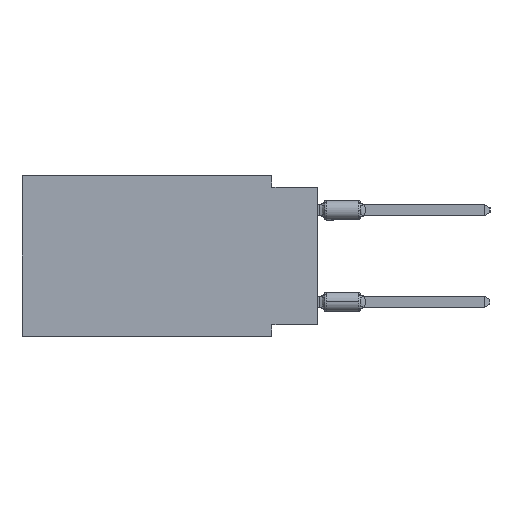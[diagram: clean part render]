
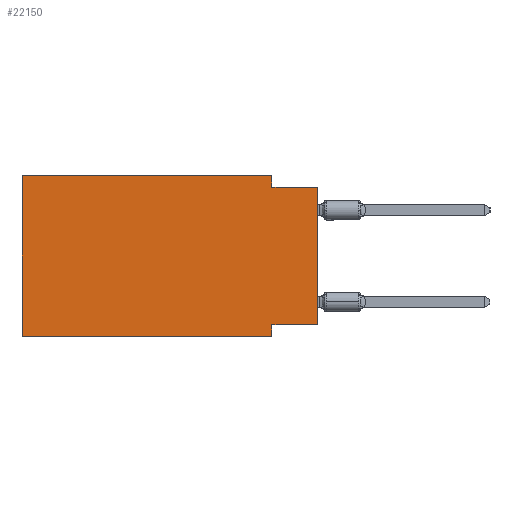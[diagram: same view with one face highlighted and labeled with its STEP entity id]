
A CAD part, left-side view. The second image highlights one B-rep face of the part: STEP entity #22150.
In plain terms, the highlighted planar face has unit normal (-1, 0, 0).
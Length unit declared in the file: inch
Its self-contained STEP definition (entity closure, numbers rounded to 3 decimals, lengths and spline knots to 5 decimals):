
#158 = ORIENTED_EDGE ( 'NONE', *, *, #56466, .F. ) ;
#306 = VECTOR ( 'NONE', #60173, 39.37008 ) ;
#511 = ORIENTED_EDGE ( 'NONE', *, *, #33676, .F. ) ;
#814 = DIRECTION ( 'NONE',  ( 0., 0., -1. ) ) ;
#1471 = VERTEX_POINT ( 'NONE', #30181 ) ;
#1937 = VECTOR ( 'NONE', #21164, 39.37008 ) ;
#1983 = CARTESIAN_POINT ( 'NONE',  ( 0., 0., -0.025 ) ) ;
#2095 = VECTOR ( 'NONE', #48235, 39.37008 ) ;
#4401 = VERTEX_POINT ( 'NONE', #27706 ) ;
#5204 = LINE ( 'NONE', #50768, #1937 ) ;
#7165 = LINE ( 'NONE', #27428, #7428 ) ;
#7428 = VECTOR ( 'NONE', #26779, 39.37008 ) ;
#8396 = CARTESIAN_POINT ( 'NONE',  ( 0., 0.645, -0.35 ) ) ;
#8616 = FACE_OUTER_BOUND ( 'NONE', #26243, .T. ) ;
#9308 = CARTESIAN_POINT ( 'NONE',  ( 0., 0.1, -0.325 ) ) ;
#11739 = CARTESIAN_POINT ( 'NONE',  ( 0., 0.1, -0.35 ) ) ;
#12294 = DIRECTION ( 'NONE',  ( 0., 0., -1. ) ) ;
#12541 = EDGE_CURVE ( 'NONE', #60988, #54172, #38979, .T. ) ;
#17719 = CARTESIAN_POINT ( 'NONE',  ( 0., 0.645, 0. ) ) ;
#18236 = LINE ( 'NONE', #63796, #39655 ) ;
#18323 = EDGE_CURVE ( 'NONE', #4401, #53427, #36437, .T. ) ;
#21164 = DIRECTION ( 'NONE',  ( 0., -1., 0. ) ) ;
#21546 = ORIENTED_EDGE ( 'NONE', *, *, #18323, .T. ) ;
#22150 = ADVANCED_FACE ( 'NONE', ( #8616 ), #28557, .F. ) ;
#23129 = VECTOR ( 'NONE', #27672, 39.37008 ) ;
#23740 = CARTESIAN_POINT ( 'NONE',  ( 0., 0.645, 0. ) ) ;
#26243 = EDGE_LOOP ( 'NONE', ( #21546, #32283, #41343, #34098, #158, #36931, #511, #52017 ) ) ;
#26779 = DIRECTION ( 'NONE',  ( 0., 1., 0. ) ) ;
#26961 = LINE ( 'NONE', #47257, #2095 ) ;
#27082 = DIRECTION ( 'NONE',  ( 0., 0., 1. ) ) ;
#27428 = CARTESIAN_POINT ( 'NONE',  ( 0., 0., -0.325 ) ) ;
#27672 = DIRECTION ( 'NONE',  ( 0., -1., 0. ) ) ;
#27706 = CARTESIAN_POINT ( 'NONE',  ( 0., 0., -0.325 ) ) ;
#28557 = PLANE ( 'NONE',  #49572 ) ;
#28885 = CARTESIAN_POINT ( 'NONE',  ( 0., 0.645, 0. ) ) ;
#29329 = CARTESIAN_POINT ( 'NONE',  ( 0., 0.1, -0.025 ) ) ;
#30181 = CARTESIAN_POINT ( 'NONE',  ( 0., 0.1, 0. ) ) ;
#30734 = LINE ( 'NONE', #46375, #46731 ) ;
#32283 = ORIENTED_EDGE ( 'NONE', *, *, #32775, .F. ) ;
#32775 = EDGE_CURVE ( 'NONE', #55610, #53427, #5204, .T. ) ;
#33571 = EDGE_CURVE ( 'NONE', #4401, #48348, #7165, .T. ) ;
#33676 = EDGE_CURVE ( 'NONE', #48348, #54172, #30734, .T. ) ;
#34098 = ORIENTED_EDGE ( 'NONE', *, *, #63225, .F. ) ;
#34799 = DIRECTION ( 'NONE',  ( 0., 0., 1. ) ) ;
#36437 = LINE ( 'NONE', #56718, #45251 ) ;
#36931 = ORIENTED_EDGE ( 'NONE', *, *, #12541, .T. ) ;
#38487 = VERTEX_POINT ( 'NONE', #23740 ) ;
#38979 = LINE ( 'NONE', #8396, #306 ) ;
#39655 = VECTOR ( 'NONE', #34799, 39.37008 ) ;
#41343 = ORIENTED_EDGE ( 'NONE', *, *, #48139, .F. ) ;
#42969 = LINE ( 'NONE', #17719, #23129 ) ;
#45251 = VECTOR ( 'NONE', #27082, 39.37008 ) ;
#46375 = CARTESIAN_POINT ( 'NONE',  ( 0., 0.1, -0.35 ) ) ;
#46731 = VECTOR ( 'NONE', #814, 39.37008 ) ;
#47257 = CARTESIAN_POINT ( 'NONE',  ( 0., 0.1, 0. ) ) ;
#48139 = EDGE_CURVE ( 'NONE', #1471, #55610, #26961, .T. ) ;
#48235 = DIRECTION ( 'NONE',  ( 0., 0., -1. ) ) ;
#48348 = VERTEX_POINT ( 'NONE', #9308 ) ;
#48945 = CARTESIAN_POINT ( 'NONE',  ( 0., 0.645, -0.35 ) ) ;
#49179 = DIRECTION ( 'NONE',  ( 1., 0., 0. ) ) ;
#49572 = AXIS2_PLACEMENT_3D ( 'NONE', #28885, #49179, #12294 ) ;
#50768 = CARTESIAN_POINT ( 'NONE',  ( 0., 0., -0.025 ) ) ;
#52017 = ORIENTED_EDGE ( 'NONE', *, *, #33571, .F. ) ;
#53427 = VERTEX_POINT ( 'NONE', #1983 ) ;
#54172 = VERTEX_POINT ( 'NONE', #11739 ) ;
#55610 = VERTEX_POINT ( 'NONE', #29329 ) ;
#56466 = EDGE_CURVE ( 'NONE', #60988, #38487, #18236, .T. ) ;
#56718 = CARTESIAN_POINT ( 'NONE',  ( 0., 0., 0. ) ) ;
#60173 = DIRECTION ( 'NONE',  ( 0., -1., 0. ) ) ;
#60988 = VERTEX_POINT ( 'NONE', #48945 ) ;
#63225 = EDGE_CURVE ( 'NONE', #38487, #1471, #42969, .T. ) ;
#63796 = CARTESIAN_POINT ( 'NONE',  ( 0., 0.645, 0. ) ) ;
